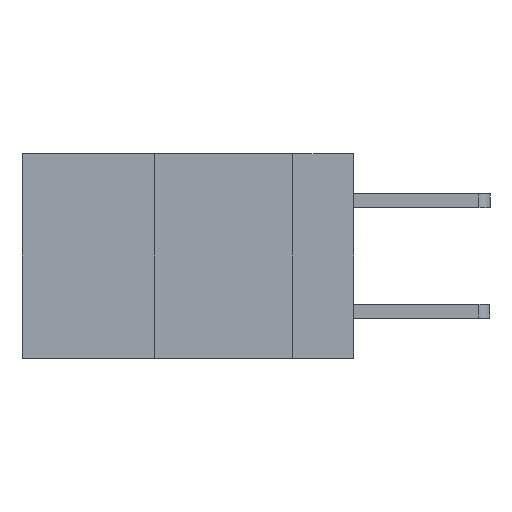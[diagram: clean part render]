
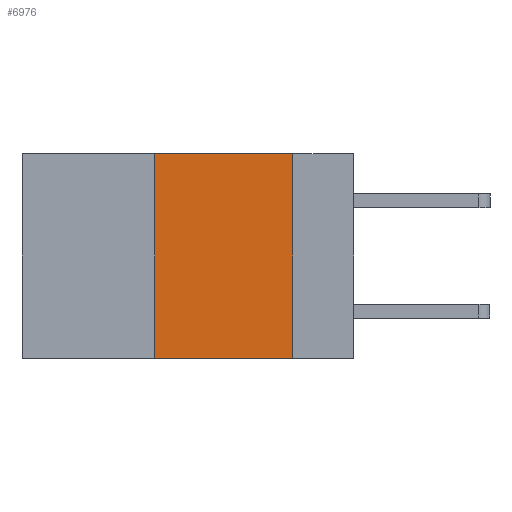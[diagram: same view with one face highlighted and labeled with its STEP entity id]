
A CAD part, left-side view. The second image highlights one B-rep face of the part: STEP entity #6976.
In plain terms, the highlighted planar face has unit normal (-1, 0, 0).
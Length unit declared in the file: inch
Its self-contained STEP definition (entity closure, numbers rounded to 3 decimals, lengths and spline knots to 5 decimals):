
#331 = LINE ( 'NONE', #9436, #2308 ) ;
#809 = ORIENTED_EDGE ( 'NONE', *, *, #3785, .F. ) ;
#885 = CARTESIAN_POINT ( 'NONE',  ( 0., 0.36, 0. ) ) ;
#1184 = ORIENTED_EDGE ( 'NONE', *, *, #10553, .F. ) ;
#1271 = FACE_OUTER_BOUND ( 'NONE', #7903, .T. ) ;
#1679 = VERTEX_POINT ( 'NONE', #10654 ) ;
#2071 = DIRECTION ( 'NONE',  ( 0., 0., -1. ) ) ;
#2308 = VECTOR ( 'NONE', #2071, 39.37008 ) ;
#2321 = CARTESIAN_POINT ( 'NONE',  ( 0., 0.11, -0.37 ) ) ;
#3217 = CARTESIAN_POINT ( 'NONE',  ( 0., 0.6, 0. ) ) ;
#3617 = EDGE_CURVE ( 'NONE', #8978, #6830, #6824, .T. ) ;
#3728 = VERTEX_POINT ( 'NONE', #2321 ) ;
#3785 = EDGE_CURVE ( 'NONE', #6830, #1679, #5639, .T. ) ;
#4666 = PLANE ( 'NONE',  #10896 ) ;
#5109 = DIRECTION ( 'NONE',  ( 0., 0., 1. ) ) ;
#5639 = LINE ( 'NONE', #3217, #7684 ) ;
#6410 = CARTESIAN_POINT ( 'NONE',  ( 0., 0.6, -0.37 ) ) ;
#6824 = LINE ( 'NONE', #885, #10315 ) ;
#6830 = VERTEX_POINT ( 'NONE', #8706 ) ;
#6976 = ADVANCED_FACE ( 'NONE', ( #1271 ), #4666, .F. ) ;
#7206 = DIRECTION ( 'NONE',  ( 1., 0., 0. ) ) ;
#7663 = EDGE_CURVE ( 'NONE', #8978, #3728, #8170, .T. ) ;
#7684 = VECTOR ( 'NONE', #9945, 39.37008 ) ;
#7903 = EDGE_LOOP ( 'NONE', ( #1184, #809, #10270, #8980 ) ) ;
#7905 = VECTOR ( 'NONE', #8285, 39.37008 ) ;
#8026 = CARTESIAN_POINT ( 'NONE',  ( 0., 0.6, 0. ) ) ;
#8170 = LINE ( 'NONE', #6410, #7905 ) ;
#8285 = DIRECTION ( 'NONE',  ( 0., -1., 0. ) ) ;
#8706 = CARTESIAN_POINT ( 'NONE',  ( 0., 0.36, 0. ) ) ;
#8978 = VERTEX_POINT ( 'NONE', #10534 ) ;
#8980 = ORIENTED_EDGE ( 'NONE', *, *, #7663, .T. ) ;
#9436 = CARTESIAN_POINT ( 'NONE',  ( 0., 0.11, 0. ) ) ;
#9735 = DIRECTION ( 'NONE',  ( 0., 0., -1. ) ) ;
#9945 = DIRECTION ( 'NONE',  ( 0., -1., 0. ) ) ;
#10270 = ORIENTED_EDGE ( 'NONE', *, *, #3617, .F. ) ;
#10315 = VECTOR ( 'NONE', #5109, 39.37008 ) ;
#10534 = CARTESIAN_POINT ( 'NONE',  ( 0., 0.36, -0.37 ) ) ;
#10553 = EDGE_CURVE ( 'NONE', #1679, #3728, #331, .T. ) ;
#10654 = CARTESIAN_POINT ( 'NONE',  ( 0., 0.11, 0. ) ) ;
#10896 = AXIS2_PLACEMENT_3D ( 'NONE', #8026, #7206, #9735 ) ;
